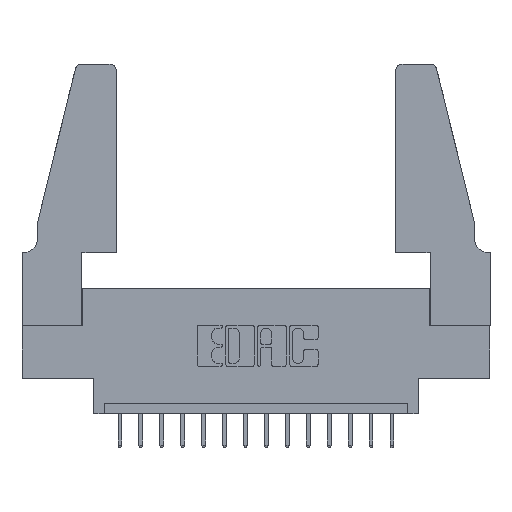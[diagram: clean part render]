
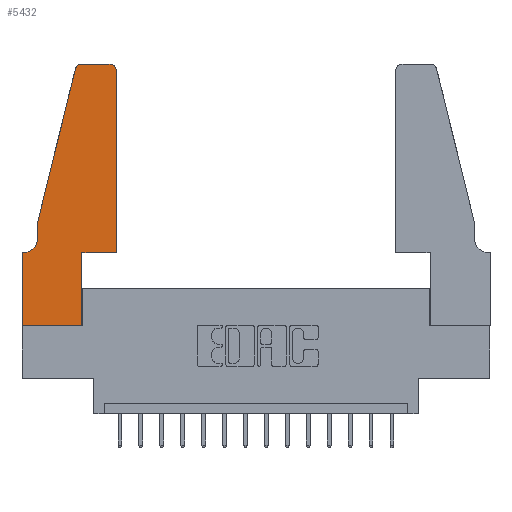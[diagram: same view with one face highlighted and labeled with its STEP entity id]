
A CAD part, top view. The second image highlights one B-rep face of the part: STEP entity #5432.
In plain terms, the highlighted planar face has unit normal (0, 0, 1).
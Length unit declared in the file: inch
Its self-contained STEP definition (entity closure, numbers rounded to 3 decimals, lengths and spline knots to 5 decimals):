
#98 = ORIENTED_EDGE ( 'NONE', *, *, #14316, .T. ) ;
#257 = LINE ( 'NONE', #9930, #10112 ) ;
#306 = VECTOR ( 'NONE', #11567, 39.37008 ) ;
#475 = DIRECTION ( 'NONE',  ( 0., 0., 1. ) ) ;
#649 = EDGE_CURVE ( 'NONE', #10471, #12002, #6417, .T. ) ;
#1137 = DIRECTION ( 'NONE',  ( -1., 0., 0. ) ) ;
#1391 = EDGE_LOOP ( 'NONE', ( #13826, #9198, #2860, #9436, #10453, #1926, #98, #5326, #15572, #7827, #2723, #8814 ) ) ;
#1504 = VECTOR ( 'NONE', #9408, 39.37008 ) ;
#1558 = CARTESIAN_POINT ( 'NONE',  ( 0.4205, 1.22, 0.37 ) ) ;
#1926 = ORIENTED_EDGE ( 'NONE', *, *, #5406, .T. ) ;
#2241 = CARTESIAN_POINT ( 'NONE',  ( 0.4505, 0.35, 0.37 ) ) ;
#2349 = CARTESIAN_POINT ( 'NONE',  ( 0.0055, 0.42, 0.37 ) ) ;
#2370 = EDGE_CURVE ( 'NONE', #9337, #14730, #12607, .T. ) ;
#2390 = EDGE_CURVE ( 'NONE', #12002, #12236, #4832, .T. ) ;
#2723 = ORIENTED_EDGE ( 'NONE', *, *, #2370, .T. ) ;
#2779 = DIRECTION ( 'NONE',  ( -0.239, -0.971, 0. ) ) ;
#2860 = ORIENTED_EDGE ( 'NONE', *, *, #649, .T. ) ;
#2941 = CARTESIAN_POINT ( 'NONE',  ( 0.4505, 1.22, 0.37 ) ) ;
#3149 = EDGE_CURVE ( 'NONE', #12236, #6742, #12389, .T. ) ;
#3702 = VERTEX_POINT ( 'NONE', #4658 ) ;
#3819 = DIRECTION ( 'NONE',  ( 0., 0., -1. ) ) ;
#4021 = CARTESIAN_POINT ( 'NONE',  ( 0.0755, 0.5, 0.37 ) ) ;
#4049 = EDGE_CURVE ( 'NONE', #16196, #9337, #6179, .T. ) ;
#4501 = CARTESIAN_POINT ( 'NONE',  ( 0.0755, 0.5, 0.37 ) ) ;
#4658 = CARTESIAN_POINT ( 'NONE',  ( 0.284, 1.25, 0.37 ) ) ;
#4677 = AXIS2_PLACEMENT_3D ( 'NONE', #1558, #8174, #5526 ) ;
#4789 = VERTEX_POINT ( 'NONE', #13459 ) ;
#4832 = LINE ( 'NONE', #4501, #5414 ) ;
#4988 = CARTESIAN_POINT ( 'NONE',  ( 0.4505, 0.35, 0.37 ) ) ;
#5088 = AXIS2_PLACEMENT_3D ( 'NONE', #14538, #475, #9519 ) ;
#5103 = EDGE_CURVE ( 'NONE', #4789, #16196, #257, .T. ) ;
#5326 = ORIENTED_EDGE ( 'NONE', *, *, #14785, .T. ) ;
#5406 = EDGE_CURVE ( 'NONE', #6742, #5881, #15566, .T. ) ;
#5414 = VECTOR ( 'NONE', #9431, 39.37008 ) ;
#5432 = ADVANCED_FACE ( 'NONE', ( #9306 ), #12053, .T. ) ;
#5526 = DIRECTION ( 'NONE',  ( 1., 0., 0. ) ) ;
#5881 = VERTEX_POINT ( 'NONE', #12760 ) ;
#6179 = LINE ( 'NONE', #4988, #306 ) ;
#6417 = LINE ( 'NONE', #4021, #15266 ) ;
#6742 = VERTEX_POINT ( 'NONE', #9656 ) ;
#6963 = AXIS2_PLACEMENT_3D ( 'NONE', #2349, #3819, #1137 ) ;
#7136 = DIRECTION ( 'NONE',  ( 1., 0., 0. ) ) ;
#7221 = VECTOR ( 'NONE', #13373, 39.37008 ) ;
#7261 = EDGE_CURVE ( 'NONE', #14730, #10062, #12639, .T. ) ;
#7794 = DIRECTION ( 'NONE',  ( -1., 0., 0. ) ) ;
#7827 = ORIENTED_EDGE ( 'NONE', *, *, #4049, .T. ) ;
#8003 = EDGE_CURVE ( 'NONE', #3702, #10471, #13020, .T. ) ;
#8030 = DIRECTION ( 'NONE',  ( 0., 1., 0. ) ) ;
#8174 = DIRECTION ( 'NONE',  ( 0., 0., 1. ) ) ;
#8724 = CARTESIAN_POINT ( 'NONE',  ( 0.4205, 1.25, 0.37 ) ) ;
#8814 = ORIENTED_EDGE ( 'NONE', *, *, #7261, .T. ) ;
#9198 = ORIENTED_EDGE ( 'NONE', *, *, #8003, .T. ) ;
#9306 = FACE_OUTER_BOUND ( 'NONE', #1391, .T. ) ;
#9337 = VERTEX_POINT ( 'NONE', #2241 ) ;
#9408 = DIRECTION ( 'NONE',  ( 0., -1., 0. ) ) ;
#9431 = DIRECTION ( 'NONE',  ( 0., -1., 0. ) ) ;
#9436 = ORIENTED_EDGE ( 'NONE', *, *, #2390, .T. ) ;
#9519 = DIRECTION ( 'NONE',  ( 1., 0., 0. ) ) ;
#9656 = CARTESIAN_POINT ( 'NONE',  ( 0.0055, 0.35, 0.37 ) ) ;
#9930 = CARTESIAN_POINT ( 'NONE',  ( 0.2865, 0.35, 0.37 ) ) ;
#10062 = VERTEX_POINT ( 'NONE', #8724 ) ;
#10112 = VECTOR ( 'NONE', #8030, 39.37008 ) ;
#10307 = CARTESIAN_POINT ( 'NONE',  ( 0.0755, 0.35, 0.37 ) ) ;
#10379 = CARTESIAN_POINT ( 'NONE',  ( 0.2605, 1.25, 0.37 ) ) ;
#10393 = CARTESIAN_POINT ( 'NONE',  ( 0.0755, 0.5, 0.37 ) ) ;
#10453 = ORIENTED_EDGE ( 'NONE', *, *, #3149, .T. ) ;
#10471 = VERTEX_POINT ( 'NONE', #13205 ) ;
#10885 = DIRECTION ( 'NONE',  ( 1., 0., 0. ) ) ;
#10947 = VECTOR ( 'NONE', #15417, 39.37008 ) ;
#11040 = CARTESIAN_POINT ( 'NONE',  ( 0.284, 1.22, 0.37 ) ) ;
#11097 = DIRECTION ( 'NONE',  ( 0., 0., 1. ) ) ;
#11412 = VECTOR ( 'NONE', #10885, 39.37008 ) ;
#11567 = DIRECTION ( 'NONE',  ( 1., 0., 0. ) ) ;
#12002 = VERTEX_POINT ( 'NONE', #10393 ) ;
#12053 = PLANE ( 'NONE',  #5088 ) ;
#12236 = VERTEX_POINT ( 'NONE', #14922 ) ;
#12371 = LINE ( 'NONE', #14779, #1504 ) ;
#12389 = CIRCLE ( 'NONE', #6963, 0.07 ) ;
#12530 = EDGE_CURVE ( 'NONE', #10062, #3702, #14777, .T. ) ;
#12607 = LINE ( 'NONE', #14802, #7221 ) ;
#12639 = CIRCLE ( 'NONE', #4677, 0.03 ) ;
#12760 = CARTESIAN_POINT ( 'NONE',  ( 0., 0.35, 0.37 ) ) ;
#12898 = AXIS2_PLACEMENT_3D ( 'NONE', #11040, #11097, #7136 ) ;
#13020 = CIRCLE ( 'NONE', #12898, 0.03 ) ;
#13205 = CARTESIAN_POINT ( 'NONE',  ( 0.25487, 1.22718, 0.37 ) ) ;
#13373 = DIRECTION ( 'NONE',  ( 0., 1., 0. ) ) ;
#13459 = CARTESIAN_POINT ( 'NONE',  ( 0.2865, 0., 0.37 ) ) ;
#13747 = VECTOR ( 'NONE', #7794, 39.37008 ) ;
#13826 = ORIENTED_EDGE ( 'NONE', *, *, #12530, .T. ) ;
#14228 = LINE ( 'NONE', #14830, #11412 ) ;
#14264 = VERTEX_POINT ( 'NONE', #14376 ) ;
#14316 = EDGE_CURVE ( 'NONE', #5881, #14264, #12371, .T. ) ;
#14376 = CARTESIAN_POINT ( 'NONE',  ( 0., 0., 0.37 ) ) ;
#14538 = CARTESIAN_POINT ( 'NONE',  ( 0., 0.35, 0.37 ) ) ;
#14725 = CARTESIAN_POINT ( 'NONE',  ( 0.2865, 0.35, 0.37 ) ) ;
#14730 = VERTEX_POINT ( 'NONE', #2941 ) ;
#14777 = LINE ( 'NONE', #10379, #10947 ) ;
#14779 = CARTESIAN_POINT ( 'NONE',  ( 0., 0., 0.37 ) ) ;
#14785 = EDGE_CURVE ( 'NONE', #14264, #4789, #14228, .T. ) ;
#14802 = CARTESIAN_POINT ( 'NONE',  ( 0.4505, 0.35, 0.37 ) ) ;
#14830 = CARTESIAN_POINT ( 'NONE',  ( 0., 0., 0.37 ) ) ;
#14922 = CARTESIAN_POINT ( 'NONE',  ( 0.0755, 0.42, 0.37 ) ) ;
#15266 = VECTOR ( 'NONE', #2779, 39.37008 ) ;
#15417 = DIRECTION ( 'NONE',  ( -1., 0., 0. ) ) ;
#15566 = LINE ( 'NONE', #10307, #13747 ) ;
#15572 = ORIENTED_EDGE ( 'NONE', *, *, #5103, .T. ) ;
#16196 = VERTEX_POINT ( 'NONE', #14725 ) ;
